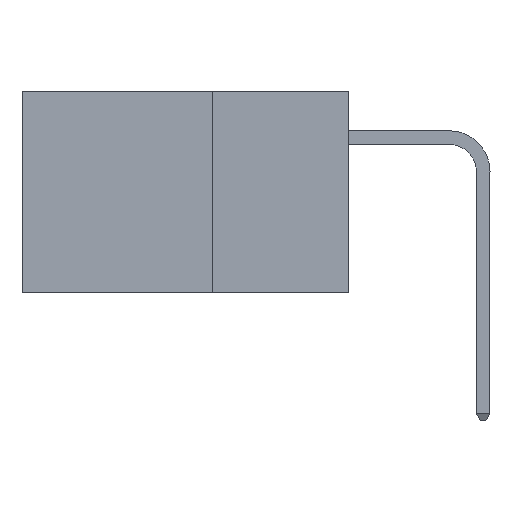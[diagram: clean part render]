
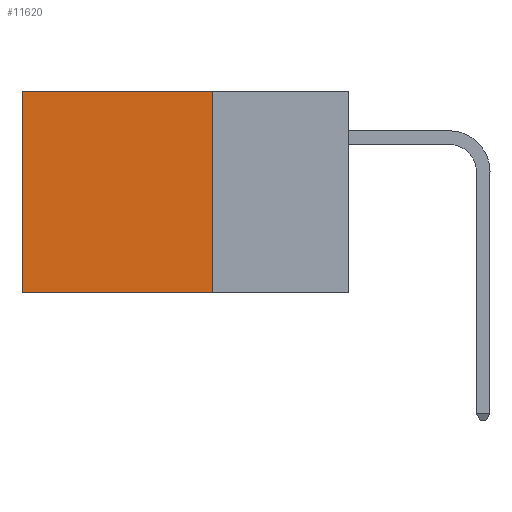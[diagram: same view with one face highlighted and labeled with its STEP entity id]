
A CAD part, left-side view. The second image highlights one B-rep face of the part: STEP entity #11620.
In plain terms, the highlighted planar face has unit normal (-1, 0, 0).
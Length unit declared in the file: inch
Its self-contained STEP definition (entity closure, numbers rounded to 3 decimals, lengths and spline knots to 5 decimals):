
#514 = VECTOR ( 'NONE', #14032, 39.37008 ) ;
#582 = ORIENTED_EDGE ( 'NONE', *, *, #17358, .F. ) ;
#749 = PLANE ( 'NONE',  #11758 ) ;
#1568 = CARTESIAN_POINT ( 'NONE',  ( 0.2875, 0.25, 0. ) ) ;
#1774 = LINE ( 'NONE', #1568, #20091 ) ;
#2838 = LINE ( 'NONE', #2841, #11772 ) ;
#2840 = VECTOR ( 'NONE', #15253, 39.37008 ) ;
#2841 = CARTESIAN_POINT ( 'NONE',  ( 0.2875, 0.6, 0. ) ) ;
#3372 = CARTESIAN_POINT ( 'NONE',  ( 0.2875, 0.25, -0.37 ) ) ;
#3974 = EDGE_LOOP ( 'NONE', ( #16059, #582, #7164, #9420 ) ) ;
#4637 = DIRECTION ( 'NONE',  ( 0., 0., -1. ) ) ;
#5992 = VERTEX_POINT ( 'NONE', #15580 ) ;
#6066 = EDGE_CURVE ( 'NONE', #19527, #6829, #1774, .T. ) ;
#6202 = CARTESIAN_POINT ( 'NONE',  ( 0.2875, 0.6, 0. ) ) ;
#6829 = VERTEX_POINT ( 'NONE', #6202 ) ;
#7164 = ORIENTED_EDGE ( 'NONE', *, *, #7496, .F. ) ;
#7496 = EDGE_CURVE ( 'NONE', #19527, #9626, #17010, .T. ) ;
#7673 = FACE_OUTER_BOUND ( 'NONE', #3974, .T. ) ;
#9420 = ORIENTED_EDGE ( 'NONE', *, *, #6066, .T. ) ;
#9626 = VERTEX_POINT ( 'NONE', #16345 ) ;
#11490 = DIRECTION ( 'NONE',  ( 0., 0., -1. ) ) ;
#11620 = ADVANCED_FACE ( 'NONE', ( #7673 ), #749, .F. ) ;
#11758 = AXIS2_PLACEMENT_3D ( 'NONE', #18511, #22071, #11490 ) ;
#11772 = VECTOR ( 'NONE', #4637, 39.37008 ) ;
#14032 = DIRECTION ( 'NONE',  ( 0., 1., 0. ) ) ;
#14040 = DIRECTION ( 'NONE',  ( 0., 1., 0. ) ) ;
#14145 = LINE ( 'NONE', #3372, #514 ) ;
#15253 = DIRECTION ( 'NONE',  ( 0., 0., -1. ) ) ;
#15580 = CARTESIAN_POINT ( 'NONE',  ( 0.2875, 0.6, -0.37 ) ) ;
#15588 = CARTESIAN_POINT ( 'NONE',  ( 0.2875, 0.25, 0. ) ) ;
#16059 = ORIENTED_EDGE ( 'NONE', *, *, #22537, .T. ) ;
#16345 = CARTESIAN_POINT ( 'NONE',  ( 0.2875, 0.25, -0.37 ) ) ;
#17010 = LINE ( 'NONE', #18696, #2840 ) ;
#17358 = EDGE_CURVE ( 'NONE', #9626, #5992, #14145, .T. ) ;
#18511 = CARTESIAN_POINT ( 'NONE',  ( 0.2875, 0.25, 0. ) ) ;
#18696 = CARTESIAN_POINT ( 'NONE',  ( 0.2875, 0.25, 0. ) ) ;
#19527 = VERTEX_POINT ( 'NONE', #15588 ) ;
#20091 = VECTOR ( 'NONE', #14040, 39.37008 ) ;
#22071 = DIRECTION ( 'NONE',  ( 1., 0., 0. ) ) ;
#22537 = EDGE_CURVE ( 'NONE', #6829, #5992, #2838, .T. ) ;
